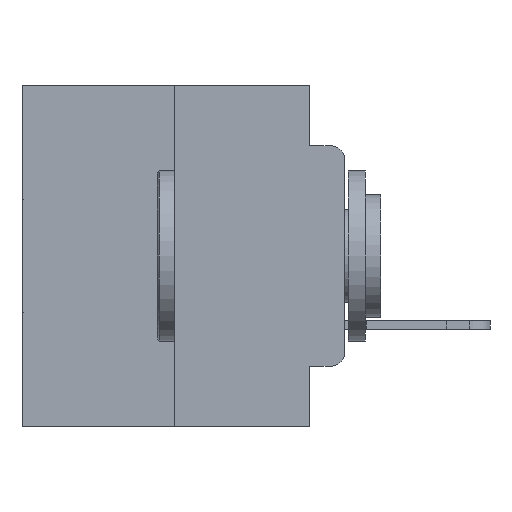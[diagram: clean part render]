
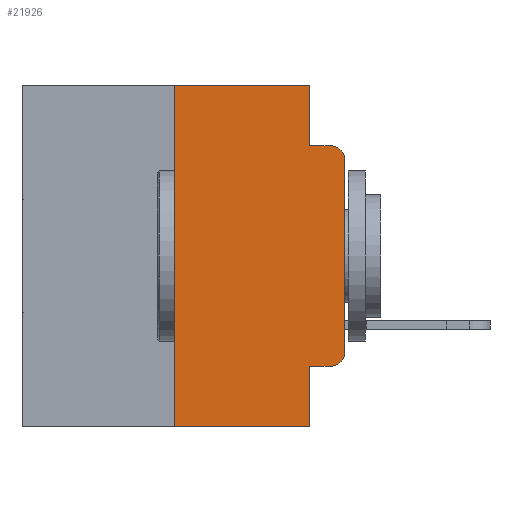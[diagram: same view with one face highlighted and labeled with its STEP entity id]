
A CAD part, left-side view. The second image highlights one B-rep face of the part: STEP entity #21926.
In plain terms, the highlighted planar face has unit normal (-1, 0, 0).
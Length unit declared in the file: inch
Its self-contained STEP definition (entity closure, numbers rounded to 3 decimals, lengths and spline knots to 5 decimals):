
#246 = CARTESIAN_POINT ( 'NONE',  ( 0., 0., -0.1085 ) ) ;
#308 = VECTOR ( 'NONE', #23043, 39.37008 ) ;
#667 = DIRECTION ( 'NONE',  ( 0., 0., -1. ) ) ;
#1915 = AXIS2_PLACEMENT_3D ( 'NONE', #27718, #7745, #667 ) ;
#2126 = EDGE_CURVE ( 'NONE', #15713, #25696, #13738, .T. ) ;
#2291 = CARTESIAN_POINT ( 'NONE',  ( 0., 0.02, -0.0885 ) ) ;
#2600 = CARTESIAN_POINT ( 'NONE',  ( 0., 0., -0.3915 ) ) ;
#3322 = EDGE_CURVE ( 'NONE', #3814, #17626, #3511, .T. ) ;
#3484 = VERTEX_POINT ( 'NONE', #9343 ) ;
#3511 = LINE ( 'NONE', #17921, #8063 ) ;
#3749 = EDGE_CURVE ( 'NONE', #5163, #17626, #24161, .T. ) ;
#3814 = VERTEX_POINT ( 'NONE', #21614 ) ;
#4323 = VERTEX_POINT ( 'NONE', #2291 ) ;
#4387 = EDGE_CURVE ( 'NONE', #5163, #15547, #23423, .T. ) ;
#4554 = EDGE_CURVE ( 'NONE', #15547, #15713, #12164, .T. ) ;
#4783 = EDGE_CURVE ( 'NONE', #8294, #20282, #14240, .T. ) ;
#4967 = ORIENTED_EDGE ( 'NONE', *, *, #21732, .F. ) ;
#5109 = ORIENTED_EDGE ( 'NONE', *, *, #3322, .T. ) ;
#5163 = VERTEX_POINT ( 'NONE', #21655 ) ;
#5614 = CARTESIAN_POINT ( 'NONE',  ( 0., 0.051, 0. ) ) ;
#5672 = VECTOR ( 'NONE', #18391, 39.37008 ) ;
#5840 = VECTOR ( 'NONE', #28800, 39.37008 ) ;
#6210 = AXIS2_PLACEMENT_3D ( 'NONE', #12020, #9753, #12419 ) ;
#6261 = CARTESIAN_POINT ( 'NONE',  ( 0., 0.051, 0. ) ) ;
#6292 = EDGE_LOOP ( 'NONE', ( #10087, #28619, #13042, #4967, #24816, #26422, #5109, #9284, #27562, #8046 ) ) ;
#7360 = CARTESIAN_POINT ( 'NONE',  ( 0., 0.051, 0. ) ) ;
#7745 = DIRECTION ( 'NONE',  ( -1., 0., 0. ) ) ;
#8046 = ORIENTED_EDGE ( 'NONE', *, *, #4554, .T. ) ;
#8063 = VECTOR ( 'NONE', #24669, 39.37008 ) ;
#8294 = VERTEX_POINT ( 'NONE', #16679 ) ;
#8704 = VECTOR ( 'NONE', #18326, 39.37008 ) ;
#8725 = CIRCLE ( 'NONE', #6210, 0.02 ) ;
#9284 = ORIENTED_EDGE ( 'NONE', *, *, #3749, .F. ) ;
#9343 = CARTESIAN_POINT ( 'NONE',  ( 0., 0.051, -0.0885 ) ) ;
#9753 = DIRECTION ( 'NONE',  ( -1., 0., 0. ) ) ;
#9950 = VECTOR ( 'NONE', #12785, 39.37008 ) ;
#10087 = ORIENTED_EDGE ( 'NONE', *, *, #2126, .T. ) ;
#10353 = LINE ( 'NONE', #7360, #308 ) ;
#10461 = CARTESIAN_POINT ( 'NONE',  ( 0., 0., 0. ) ) ;
#10726 = CARTESIAN_POINT ( 'NONE',  ( 0., 0.051, -0.0885 ) ) ;
#10781 = AXIS2_PLACEMENT_3D ( 'NONE', #28832, #15792, #22168 ) ;
#10887 = PLANE ( 'NONE',  #10781 ) ;
#11042 = CARTESIAN_POINT ( 'NONE',  ( 0., 0.051, -0.5 ) ) ;
#12020 = CARTESIAN_POINT ( 'NONE',  ( 0., 0.02, -0.1085 ) ) ;
#12164 = CIRCLE ( 'NONE', #1915, 0.02 ) ;
#12419 = DIRECTION ( 'NONE',  ( 0., 0., -1. ) ) ;
#12785 = DIRECTION ( 'NONE',  ( 0., -1., 0. ) ) ;
#13042 = ORIENTED_EDGE ( 'NONE', *, *, #13503, .F. ) ;
#13503 = EDGE_CURVE ( 'NONE', #3484, #4323, #15952, .T. ) ;
#13738 = LINE ( 'NONE', #10461, #5672 ) ;
#14240 = LINE ( 'NONE', #19799, #5840 ) ;
#15016 = DIRECTION ( 'NONE',  ( 0., 0., 1. ) ) ;
#15547 = VERTEX_POINT ( 'NONE', #22297 ) ;
#15713 = VERTEX_POINT ( 'NONE', #2600 ) ;
#15792 = DIRECTION ( 'NONE',  ( 1., 0., 0. ) ) ;
#15952 = LINE ( 'NONE', #10726, #9950 ) ;
#16679 = CARTESIAN_POINT ( 'NONE',  ( 0., 0.25, 0. ) ) ;
#17626 = VERTEX_POINT ( 'NONE', #11042 ) ;
#17921 = CARTESIAN_POINT ( 'NONE',  ( 0., 0.473, -0.5 ) ) ;
#18326 = DIRECTION ( 'NONE',  ( 0., -1., 0. ) ) ;
#18391 = DIRECTION ( 'NONE',  ( 0., 0., 1. ) ) ;
#19799 = CARTESIAN_POINT ( 'NONE',  ( 0., 0.473, 0. ) ) ;
#20282 = VERTEX_POINT ( 'NONE', #6261 ) ;
#20688 = EDGE_CURVE ( 'NONE', #25696, #4323, #8725, .T. ) ;
#21614 = CARTESIAN_POINT ( 'NONE',  ( 0., 0.25, -0.5 ) ) ;
#21655 = CARTESIAN_POINT ( 'NONE',  ( 0., 0.051, -0.4115 ) ) ;
#21732 = EDGE_CURVE ( 'NONE', #20282, #3484, #10353, .T. ) ;
#21926 = ADVANCED_FACE ( 'NONE', ( #23504 ), #10887, .F. ) ;
#22168 = DIRECTION ( 'NONE',  ( 0., 0., -1. ) ) ;
#22172 = LINE ( 'NONE', #25883, #24278 ) ;
#22297 = CARTESIAN_POINT ( 'NONE',  ( 0., 0.02, -0.4115 ) ) ;
#23043 = DIRECTION ( 'NONE',  ( 0., 0., -1. ) ) ;
#23423 = LINE ( 'NONE', #24798, #8704 ) ;
#23456 = VECTOR ( 'NONE', #25906, 39.37008 ) ;
#23504 = FACE_OUTER_BOUND ( 'NONE', #6292, .T. ) ;
#24161 = LINE ( 'NONE', #5614, #23456 ) ;
#24278 = VECTOR ( 'NONE', #15016, 39.37008 ) ;
#24669 = DIRECTION ( 'NONE',  ( 0., -1., 0. ) ) ;
#24798 = CARTESIAN_POINT ( 'NONE',  ( 0., 0.051, -0.4115 ) ) ;
#24816 = ORIENTED_EDGE ( 'NONE', *, *, #4783, .F. ) ;
#25696 = VERTEX_POINT ( 'NONE', #246 ) ;
#25883 = CARTESIAN_POINT ( 'NONE',  ( 0., 0.25, 0. ) ) ;
#25906 = DIRECTION ( 'NONE',  ( 0., 0., -1. ) ) ;
#26422 = ORIENTED_EDGE ( 'NONE', *, *, #26532, .F. ) ;
#26532 = EDGE_CURVE ( 'NONE', #3814, #8294, #22172, .T. ) ;
#27562 = ORIENTED_EDGE ( 'NONE', *, *, #4387, .T. ) ;
#27718 = CARTESIAN_POINT ( 'NONE',  ( 0., 0.02, -0.3915 ) ) ;
#28619 = ORIENTED_EDGE ( 'NONE', *, *, #20688, .T. ) ;
#28800 = DIRECTION ( 'NONE',  ( 0., -1., 0. ) ) ;
#28832 = CARTESIAN_POINT ( 'NONE',  ( 0., 0.473, 0. ) ) ;
